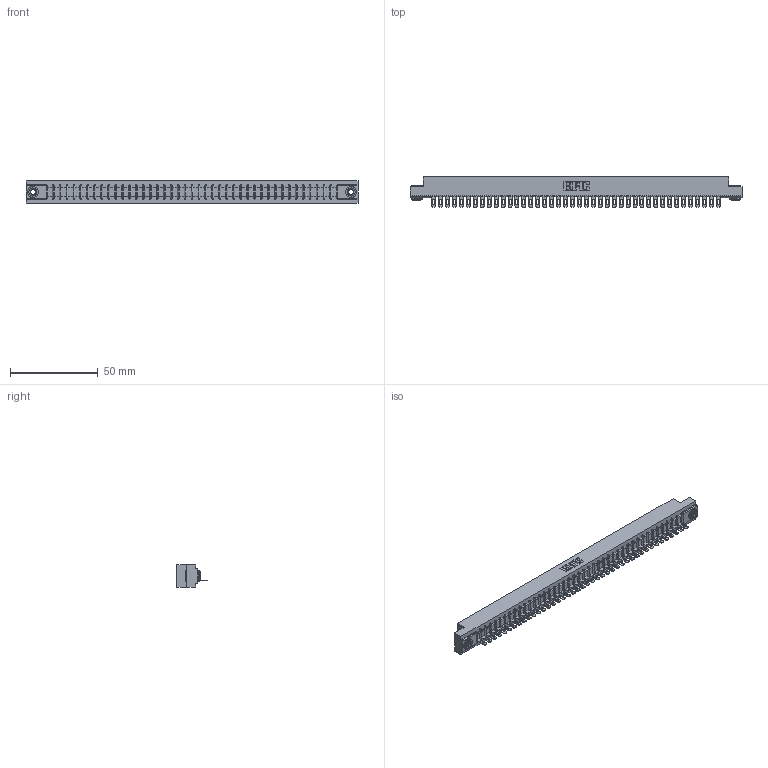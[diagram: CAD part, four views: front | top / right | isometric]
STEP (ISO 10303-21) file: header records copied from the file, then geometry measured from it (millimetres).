
FILE_DESCRIPTION (( 'STEP AP203' ), '1' );
FILE_NAME ('357-042-401-103.STEP', '2020-10-03T10:32:29', ( '' ), ( '' ), 'SwSTEP 2.0', 'SolidWorks 2020', '' );
FILE_SCHEMA (( 'CONFIG_CONTROL_DESIGN' ));
Length unit declared in the file: inch
Products named in the file (4): 307-290-002_501; 357-042-401-103; 307 Part_.156 Dia Mounting Holes; 345-250-002_345-250-002-102
Assembly tree (45 placements, depth 2):
  357-042-401-103
    307 Part_.156 Dia Mounting Holes
    307-290-002_501  x42
    345-250-002_345-250-002-102  x2
Bounding box: 189.43 x 17.42 x 12.7 mm (x, y, z)
Volume: 20309.6 mm3; surface area: 26069.3 mm2
Topology: 45 solids, 45 shells, 3405 faces, 10431 edges, 6834 vertices
Faces by surface type: plane 1942, cylinder 1369, sphere 86, cone 8
Entity records: 37865 total; most frequent: CARTESIAN_POINT 6365, ORIENTED_EDGE 6346, DIRECTION 6203, EDGE_CURVE 3173, VECTOR 2419, LINE 2419, VERTEX_POINT 2054, AXIS2_PLACEMENT_3D 1892
